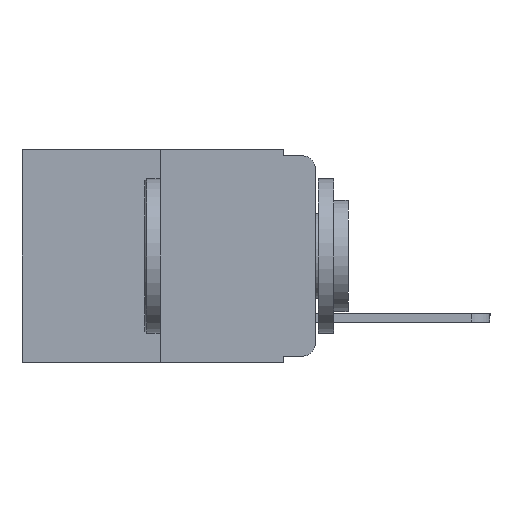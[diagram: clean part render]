
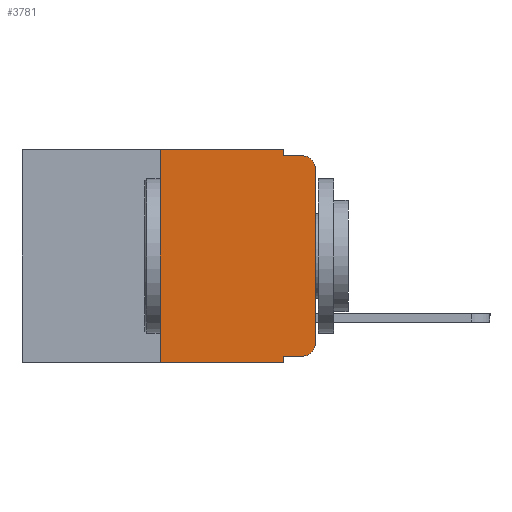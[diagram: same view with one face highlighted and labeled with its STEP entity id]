
A CAD part, left-side view. The second image highlights one B-rep face of the part: STEP entity #3781.
In plain terms, the highlighted planar face has unit normal (-1, 0, 0).
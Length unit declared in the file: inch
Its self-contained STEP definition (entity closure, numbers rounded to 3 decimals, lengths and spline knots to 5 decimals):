
#220 = DIRECTION ( 'NONE',  ( 0., 0., -1. ) ) ;
#228 = DIRECTION ( 'NONE',  ( 0., -1., 0. ) ) ;
#459 = DIRECTION ( 'NONE',  ( 0., -1., 0. ) ) ;
#500 = AXIS2_PLACEMENT_3D ( 'NONE', #2715, #13262, #4410 ) ;
#849 = ORIENTED_EDGE ( 'NONE', *, *, #16530, .F. ) ;
#883 = CARTESIAN_POINT ( 'NONE',  ( 0., 0.051, 0. ) ) ;
#915 = CARTESIAN_POINT ( 'NONE',  ( 0., 0.25, 0. ) ) ;
#1014 = PLANE ( 'NONE',  #500 ) ;
#1115 = VECTOR ( 'NONE', #18992, 39.37008 ) ;
#1378 = CIRCLE ( 'NONE', #18435, 0.02 ) ;
#1402 = DIRECTION ( 'NONE',  ( 0., -1., 0. ) ) ;
#1891 = ORIENTED_EDGE ( 'NONE', *, *, #16497, .T. ) ;
#2093 = VECTOR ( 'NONE', #12521, 39.37008 ) ;
#2139 = DIRECTION ( 'NONE',  ( 0., -1., 0. ) ) ;
#2638 = VERTEX_POINT ( 'NONE', #883 ) ;
#2715 = CARTESIAN_POINT ( 'NONE',  ( 0., 0.473, 0. ) ) ;
#3582 = EDGE_CURVE ( 'NONE', #10615, #2638, #8010, .T. ) ;
#3752 = ORIENTED_EDGE ( 'NONE', *, *, #16231, .T. ) ;
#3781 = ADVANCED_FACE ( 'NONE', ( #18541 ), #1014, .F. ) ;
#3789 = VECTOR ( 'NONE', #1402, 39.37008 ) ;
#4410 = DIRECTION ( 'NONE',  ( 0., 0., -1. ) ) ;
#4790 = CARTESIAN_POINT ( 'NONE',  ( 0., 0.051, -0.01 ) ) ;
#4799 = VECTOR ( 'NONE', #220, 39.37008 ) ;
#5106 = AXIS2_PLACEMENT_3D ( 'NONE', #17392, #8949, #18758 ) ;
#5259 = CARTESIAN_POINT ( 'NONE',  ( 0., 0.473, 0. ) ) ;
#5754 = EDGE_CURVE ( 'NONE', #7421, #15080, #7973, .T. ) ;
#6488 = LINE ( 'NONE', #11086, #2093 ) ;
#7421 = VERTEX_POINT ( 'NONE', #18265 ) ;
#7540 = CARTESIAN_POINT ( 'NONE',  ( 0., 0., -0.03 ) ) ;
#7781 = CARTESIAN_POINT ( 'NONE',  ( 0., 0., 0. ) ) ;
#7973 = LINE ( 'NONE', #4790, #3789 ) ;
#7984 = VERTEX_POINT ( 'NONE', #11363 ) ;
#8010 = LINE ( 'NONE', #5259, #15111 ) ;
#8201 = CARTESIAN_POINT ( 'NONE',  ( 0., 0.02, -0.03 ) ) ;
#8537 = VECTOR ( 'NONE', #459, 39.37008 ) ;
#8949 = DIRECTION ( 'NONE',  ( -1., 0., 0. ) ) ;
#9028 = ORIENTED_EDGE ( 'NONE', *, *, #11003, .F. ) ;
#9174 = EDGE_CURVE ( 'NONE', #2638, #7421, #10959, .T. ) ;
#9262 = LINE ( 'NONE', #9659, #4799 ) ;
#9414 = VERTEX_POINT ( 'NONE', #9919 ) ;
#9457 = CARTESIAN_POINT ( 'NONE',  ( 0., 0., -0.313 ) ) ;
#9532 = EDGE_LOOP ( 'NONE', ( #3752, #1891, #10574, #9880, #15444, #9028, #14613, #849, #14408, #16133 ) ) ;
#9560 = VERTEX_POINT ( 'NONE', #15873 ) ;
#9589 = DIRECTION ( 'NONE',  ( 0., 0., -1. ) ) ;
#9659 = CARTESIAN_POINT ( 'NONE',  ( 0., 0.051, 0. ) ) ;
#9862 = VERTEX_POINT ( 'NONE', #9457 ) ;
#9880 = ORIENTED_EDGE ( 'NONE', *, *, #9174, .F. ) ;
#9919 = CARTESIAN_POINT ( 'NONE',  ( 0., 0.051, -0.343 ) ) ;
#10574 = ORIENTED_EDGE ( 'NONE', *, *, #5754, .F. ) ;
#10615 = VERTEX_POINT ( 'NONE', #915 ) ;
#10893 = CARTESIAN_POINT ( 'NONE',  ( 0., 0.051, 0. ) ) ;
#10959 = LINE ( 'NONE', #10893, #17966 ) ;
#11003 = EDGE_CURVE ( 'NONE', #7984, #10615, #6488, .T. ) ;
#11086 = CARTESIAN_POINT ( 'NONE',  ( 0., 0.25, 0. ) ) ;
#11101 = EDGE_CURVE ( 'NONE', #9560, #11745, #16487, .T. ) ;
#11326 = CARTESIAN_POINT ( 'NONE',  ( 0., 0.473, -0.343 ) ) ;
#11363 = CARTESIAN_POINT ( 'NONE',  ( 0., 0.25, -0.343 ) ) ;
#11745 = VERTEX_POINT ( 'NONE', #12627 ) ;
#12521 = DIRECTION ( 'NONE',  ( 0., 0., 1. ) ) ;
#12627 = CARTESIAN_POINT ( 'NONE',  ( 0., 0.02, -0.333 ) ) ;
#12773 = CARTESIAN_POINT ( 'NONE',  ( 0., 0.051, -0.333 ) ) ;
#13262 = DIRECTION ( 'NONE',  ( 1., 0., 0. ) ) ;
#13488 = EDGE_CURVE ( 'NONE', #11745, #9862, #15777, .T. ) ;
#14408 = ORIENTED_EDGE ( 'NONE', *, *, #11101, .T. ) ;
#14613 = ORIENTED_EDGE ( 'NONE', *, *, #18542, .T. ) ;
#14871 = VERTEX_POINT ( 'NONE', #7540 ) ;
#15080 = VERTEX_POINT ( 'NONE', #17771 ) ;
#15111 = VECTOR ( 'NONE', #228, 39.37008 ) ;
#15444 = ORIENTED_EDGE ( 'NONE', *, *, #3582, .F. ) ;
#15777 = CIRCLE ( 'NONE', #5106, 0.02 ) ;
#15873 = CARTESIAN_POINT ( 'NONE',  ( 0., 0.051, -0.333 ) ) ;
#16133 = ORIENTED_EDGE ( 'NONE', *, *, #13488, .T. ) ;
#16231 = EDGE_CURVE ( 'NONE', #9862, #14871, #16559, .T. ) ;
#16487 = LINE ( 'NONE', #12773, #8537 ) ;
#16497 = EDGE_CURVE ( 'NONE', #14871, #15080, #1378, .T. ) ;
#16530 = EDGE_CURVE ( 'NONE', #9560, #9414, #9262, .T. ) ;
#16559 = LINE ( 'NONE', #7781, #1115 ) ;
#17392 = CARTESIAN_POINT ( 'NONE',  ( 0., 0.02, -0.313 ) ) ;
#17771 = CARTESIAN_POINT ( 'NONE',  ( 0., 0.02, -0.01 ) ) ;
#17867 = DIRECTION ( 'NONE',  ( 0., 0., -1. ) ) ;
#17966 = VECTOR ( 'NONE', #17867, 39.37008 ) ;
#18045 = DIRECTION ( 'NONE',  ( -1., 0., 0. ) ) ;
#18098 = VECTOR ( 'NONE', #2139, 39.37008 ) ;
#18265 = CARTESIAN_POINT ( 'NONE',  ( 0., 0.051, -0.01 ) ) ;
#18435 = AXIS2_PLACEMENT_3D ( 'NONE', #8201, #18045, #9589 ) ;
#18522 = LINE ( 'NONE', #11326, #18098 ) ;
#18541 = FACE_OUTER_BOUND ( 'NONE', #9532, .T. ) ;
#18542 = EDGE_CURVE ( 'NONE', #7984, #9414, #18522, .T. ) ;
#18758 = DIRECTION ( 'NONE',  ( 0., 0., -1. ) ) ;
#18992 = DIRECTION ( 'NONE',  ( 0., 0., 1. ) ) ;
